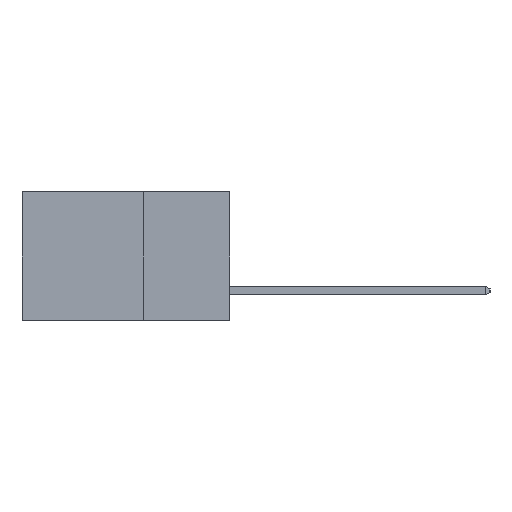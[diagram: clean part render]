
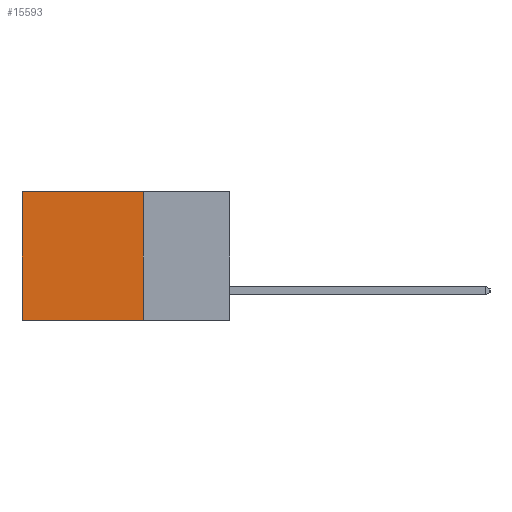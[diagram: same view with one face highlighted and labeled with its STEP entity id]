
A CAD part, left-side view. The second image highlights one B-rep face of the part: STEP entity #15593.
In plain terms, the highlighted planar face has unit normal (-1, 0, 0).
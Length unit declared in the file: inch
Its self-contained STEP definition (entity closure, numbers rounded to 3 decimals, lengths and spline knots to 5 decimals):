
#335 = VERTEX_POINT ( 'NONE', #15723 ) ;
#800 = ORIENTED_EDGE ( 'NONE', *, *, #8215, .F. ) ;
#1331 = ORIENTED_EDGE ( 'NONE', *, *, #12232, .T. ) ;
#1699 = DIRECTION ( 'NONE',  ( 0., 1., 0. ) ) ;
#2371 = CARTESIAN_POINT ( 'NONE',  ( 0.2615, 0.25, -0.37 ) ) ;
#3226 = CARTESIAN_POINT ( 'NONE',  ( 0.2615, 0.25, -0.37 ) ) ;
#4621 = ORIENTED_EDGE ( 'NONE', *, *, #5588, .T. ) ;
#4780 = LINE ( 'NONE', #9530, #11629 ) ;
#5116 = EDGE_CURVE ( 'NONE', #16032, #335, #8049, .T. ) ;
#5588 = EDGE_CURVE ( 'NONE', #10622, #335, #4780, .T. ) ;
#6251 = DIRECTION ( 'NONE',  ( 0., 1., 0. ) ) ;
#6655 = DIRECTION ( 'NONE',  ( 1., 0., 0. ) ) ;
#6755 = VECTOR ( 'NONE', #15989, 39.37008 ) ;
#6986 = VERTEX_POINT ( 'NONE', #8188 ) ;
#7097 = VECTOR ( 'NONE', #6251, 39.37008 ) ;
#7590 = CARTESIAN_POINT ( 'NONE',  ( 0.2615, 0.25, 0. ) ) ;
#7921 = ORIENTED_EDGE ( 'NONE', *, *, #5116, .F. ) ;
#8049 = LINE ( 'NONE', #10078, #11651 ) ;
#8188 = CARTESIAN_POINT ( 'NONE',  ( 0.2615, 0.25, 0. ) ) ;
#8215 = EDGE_CURVE ( 'NONE', #6986, #16032, #10845, .T. ) ;
#9530 = CARTESIAN_POINT ( 'NONE',  ( 0.2615, 0.6, -0.37 ) ) ;
#10078 = CARTESIAN_POINT ( 'NONE',  ( 0.2615, 0.25, -0.37 ) ) ;
#10622 = VERTEX_POINT ( 'NONE', #12855 ) ;
#10730 = CARTESIAN_POINT ( 'NONE',  ( 0.2615, 0.25, -0.37 ) ) ;
#10845 = LINE ( 'NONE', #10730, #6755 ) ;
#11065 = FACE_OUTER_BOUND ( 'NONE', #15494, .T. ) ;
#11629 = VECTOR ( 'NONE', #14861, 39.37008 ) ;
#11650 = AXIS2_PLACEMENT_3D ( 'NONE', #2371, #6655, #16070 ) ;
#11651 = VECTOR ( 'NONE', #1699, 39.37008 ) ;
#12232 = EDGE_CURVE ( 'NONE', #6986, #10622, #14283, .T. ) ;
#12855 = CARTESIAN_POINT ( 'NONE',  ( 0.2615, 0.6, 0. ) ) ;
#14283 = LINE ( 'NONE', #7590, #7097 ) ;
#14771 = PLANE ( 'NONE',  #11650 ) ;
#14861 = DIRECTION ( 'NONE',  ( 0., 0., -1. ) ) ;
#15494 = EDGE_LOOP ( 'NONE', ( #4621, #7921, #800, #1331 ) ) ;
#15593 = ADVANCED_FACE ( 'NONE', ( #11065 ), #14771, .F. ) ;
#15723 = CARTESIAN_POINT ( 'NONE',  ( 0.2615, 0.6, -0.37 ) ) ;
#15989 = DIRECTION ( 'NONE',  ( 0., 0., -1. ) ) ;
#16032 = VERTEX_POINT ( 'NONE', #3226 ) ;
#16070 = DIRECTION ( 'NONE',  ( 0., 0., -1. ) ) ;
